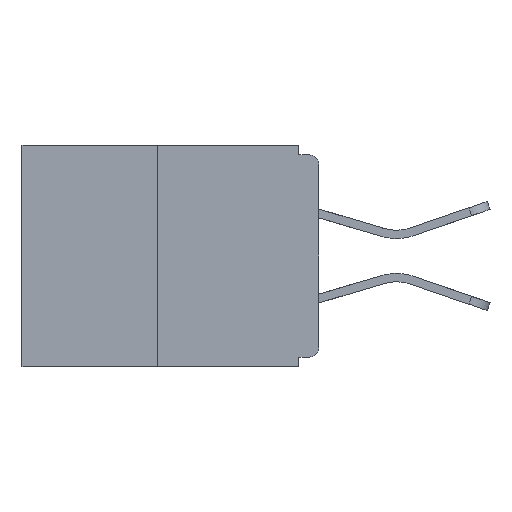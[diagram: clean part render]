
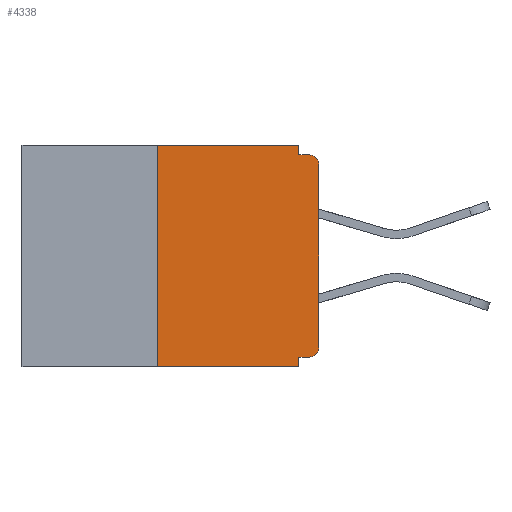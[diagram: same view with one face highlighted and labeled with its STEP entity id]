
A CAD part, left-side view. The second image highlights one B-rep face of the part: STEP entity #4338.
In plain terms, the highlighted planar face has unit normal (-1, 0, 0).
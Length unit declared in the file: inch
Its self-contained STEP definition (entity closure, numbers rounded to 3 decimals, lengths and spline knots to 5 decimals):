
#308 = CARTESIAN_POINT ( 'NONE',  ( 0., 0.46, -0.343 ) ) ;
#749 = EDGE_CURVE ( 'NONE', #2086, #5370, #8517, .T. ) ;
#948 = LINE ( 'NONE', #308, #10111 ) ;
#1023 = CARTESIAN_POINT ( 'NONE',  ( 0., 0., -0.03 ) ) ;
#1215 = LINE ( 'NONE', #15578, #5320 ) ;
#1247 = CARTESIAN_POINT ( 'NONE',  ( 0., 0.031, -0.343 ) ) ;
#1735 = CARTESIAN_POINT ( 'NONE',  ( 0., 0.46, 0. ) ) ;
#2086 = VERTEX_POINT ( 'NONE', #16765 ) ;
#2633 = VERTEX_POINT ( 'NONE', #5361 ) ;
#3099 = ORIENTED_EDGE ( 'NONE', *, *, #9429, .T. ) ;
#3623 = DIRECTION ( 'NONE',  ( 1., 0., 0. ) ) ;
#3818 = VERTEX_POINT ( 'NONE', #4757 ) ;
#4251 = VECTOR ( 'NONE', #11703, 39.37008 ) ;
#4338 = ADVANCED_FACE ( 'NONE', ( #5643 ), #8928, .F. ) ;
#4757 = CARTESIAN_POINT ( 'NONE',  ( 0., 0.031, -0.015 ) ) ;
#4791 = VERTEX_POINT ( 'NONE', #16564 ) ;
#5081 = VERTEX_POINT ( 'NONE', #17287 ) ;
#5249 = DIRECTION ( 'NONE',  ( 0., 0., -1. ) ) ;
#5320 = VECTOR ( 'NONE', #12264, 39.37008 ) ;
#5361 = CARTESIAN_POINT ( 'NONE',  ( 0., 0.25, 0. ) ) ;
#5370 = VERTEX_POINT ( 'NONE', #16892 ) ;
#5425 = EDGE_CURVE ( 'NONE', #15014, #18706, #948, .T. ) ;
#5542 = EDGE_CURVE ( 'NONE', #15014, #2633, #10917, .T. ) ;
#5611 = EDGE_CURVE ( 'NONE', #20686, #3818, #6386, .T. ) ;
#5643 = FACE_OUTER_BOUND ( 'NONE', #20035, .T. ) ;
#5894 = ORIENTED_EDGE ( 'NONE', *, *, #8891, .F. ) ;
#5955 = CIRCLE ( 'NONE', #11937, 0.015 ) ;
#6139 = LINE ( 'NONE', #8030, #21696 ) ;
#6386 = LINE ( 'NONE', #9640, #16580 ) ;
#6801 = CARTESIAN_POINT ( 'NONE',  ( 0., 0., -0.015 ) ) ;
#7218 = ORIENTED_EDGE ( 'NONE', *, *, #749, .T. ) ;
#7401 = CARTESIAN_POINT ( 'NONE',  ( 0., 0.015, -0.313 ) ) ;
#7730 = DIRECTION ( 'NONE',  ( 0., 0., -1. ) ) ;
#7758 = AXIS2_PLACEMENT_3D ( 'NONE', #7401, #14269, #19411 ) ;
#8009 = ORIENTED_EDGE ( 'NONE', *, *, #14850, .F. ) ;
#8030 = CARTESIAN_POINT ( 'NONE',  ( 0., 0., 0. ) ) ;
#8147 = CARTESIAN_POINT ( 'NONE',  ( 0., 0.031, 0. ) ) ;
#8517 = CIRCLE ( 'NONE', #7758, 0.015 ) ;
#8891 = EDGE_CURVE ( 'NONE', #2633, #20686, #18562, .T. ) ;
#8928 = PLANE ( 'NONE',  #11136 ) ;
#9117 = DIRECTION ( 'NONE',  ( 0., 0., -1. ) ) ;
#9356 = DIRECTION ( 'NONE',  ( 0., -1., 0. ) ) ;
#9429 = EDGE_CURVE ( 'NONE', #13675, #4791, #5955, .T. ) ;
#9640 = CARTESIAN_POINT ( 'NONE',  ( 0., 0.031, 0. ) ) ;
#9934 = ORIENTED_EDGE ( 'NONE', *, *, #13770, .F. ) ;
#10111 = VECTOR ( 'NONE', #9356, 39.37008 ) ;
#10151 = EDGE_CURVE ( 'NONE', #3818, #4791, #17482, .T. ) ;
#10917 = LINE ( 'NONE', #16138, #21914 ) ;
#11136 = AXIS2_PLACEMENT_3D ( 'NONE', #1735, #3623, #5249 ) ;
#11145 = DIRECTION ( 'NONE',  ( 0., 0., 1. ) ) ;
#11703 = DIRECTION ( 'NONE',  ( 0., 0., -1. ) ) ;
#11937 = AXIS2_PLACEMENT_3D ( 'NONE', #19101, #20836, #9117 ) ;
#12264 = DIRECTION ( 'NONE',  ( 0., 1., 0. ) ) ;
#12355 = VECTOR ( 'NONE', #15429, 39.37008 ) ;
#13070 = ORIENTED_EDGE ( 'NONE', *, *, #5542, .F. ) ;
#13197 = ORIENTED_EDGE ( 'NONE', *, *, #5425, .T. ) ;
#13675 = VERTEX_POINT ( 'NONE', #1023 ) ;
#13770 = EDGE_CURVE ( 'NONE', #5081, #18706, #18002, .T. ) ;
#14265 = EDGE_CURVE ( 'NONE', #5370, #13675, #6139, .T. ) ;
#14269 = DIRECTION ( 'NONE',  ( -1., 0., 0. ) ) ;
#14471 = CARTESIAN_POINT ( 'NONE',  ( 0., 0.031, -0.343 ) ) ;
#14850 = EDGE_CURVE ( 'NONE', #2086, #5081, #1215, .T. ) ;
#15014 = VERTEX_POINT ( 'NONE', #21539 ) ;
#15429 = DIRECTION ( 'NONE',  ( 0., -1., 0. ) ) ;
#15578 = CARTESIAN_POINT ( 'NONE',  ( 0., 0., -0.328 ) ) ;
#16037 = ORIENTED_EDGE ( 'NONE', *, *, #10151, .F. ) ;
#16138 = CARTESIAN_POINT ( 'NONE',  ( 0., 0.25, 0. ) ) ;
#16187 = VECTOR ( 'NONE', #21455, 39.37008 ) ;
#16440 = CARTESIAN_POINT ( 'NONE',  ( 0., 0.46, 0. ) ) ;
#16564 = CARTESIAN_POINT ( 'NONE',  ( 0., 0.015, -0.015 ) ) ;
#16580 = VECTOR ( 'NONE', #7730, 39.37008 ) ;
#16765 = CARTESIAN_POINT ( 'NONE',  ( 0., 0.015, -0.328 ) ) ;
#16892 = CARTESIAN_POINT ( 'NONE',  ( 0., 0., -0.313 ) ) ;
#17287 = CARTESIAN_POINT ( 'NONE',  ( 0., 0.031, -0.328 ) ) ;
#17482 = LINE ( 'NONE', #6801, #12355 ) ;
#18002 = LINE ( 'NONE', #1247, #4251 ) ;
#18307 = DIRECTION ( 'NONE',  ( 0., 0., 1. ) ) ;
#18562 = LINE ( 'NONE', #16440, #16187 ) ;
#18706 = VERTEX_POINT ( 'NONE', #14471 ) ;
#19101 = CARTESIAN_POINT ( 'NONE',  ( 0., 0.015, -0.03 ) ) ;
#19411 = DIRECTION ( 'NONE',  ( 0., 0., -1. ) ) ;
#20035 = EDGE_LOOP ( 'NONE', ( #5894, #13070, #13197, #9934, #8009, #7218, #20251, #3099, #16037, #21439 ) ) ;
#20251 = ORIENTED_EDGE ( 'NONE', *, *, #14265, .T. ) ;
#20686 = VERTEX_POINT ( 'NONE', #8147 ) ;
#20836 = DIRECTION ( 'NONE',  ( -1., 0., 0. ) ) ;
#21439 = ORIENTED_EDGE ( 'NONE', *, *, #5611, .F. ) ;
#21455 = DIRECTION ( 'NONE',  ( 0., -1., 0. ) ) ;
#21539 = CARTESIAN_POINT ( 'NONE',  ( 0., 0.25, -0.343 ) ) ;
#21696 = VECTOR ( 'NONE', #18307, 39.37008 ) ;
#21914 = VECTOR ( 'NONE', #11145, 39.37008 ) ;
